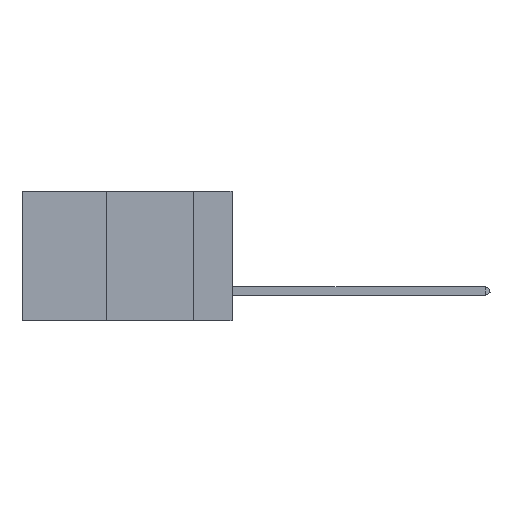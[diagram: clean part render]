
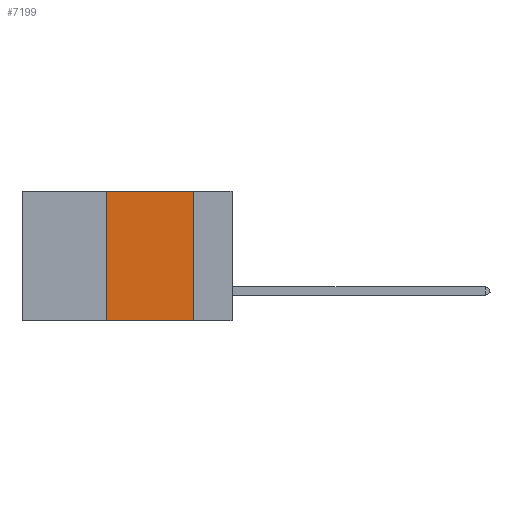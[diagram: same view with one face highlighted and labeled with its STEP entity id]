
A CAD part, left-side view. The second image highlights one B-rep face of the part: STEP entity #7199.
In plain terms, the highlighted planar face has unit normal (-1, 0, 0).
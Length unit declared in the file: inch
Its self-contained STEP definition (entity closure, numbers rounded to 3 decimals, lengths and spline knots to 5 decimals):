
#320 = CARTESIAN_POINT ( 'NONE',  ( 0., 0.36, -0.37 ) ) ;
#374 = PLANE ( 'NONE',  #565 ) ;
#406 = EDGE_CURVE ( 'NONE', #9593, #12803, #15232, .T. ) ;
#565 = AXIS2_PLACEMENT_3D ( 'NONE', #4045, #9053, #6343 ) ;
#1202 = LINE ( 'NONE', #9363, #12436 ) ;
#2927 = VECTOR ( 'NONE', #4506, 39.37008 ) ;
#2974 = EDGE_CURVE ( 'NONE', #14182, #14247, #10661, .T. ) ;
#3828 = ORIENTED_EDGE ( 'NONE', *, *, #2974, .T. ) ;
#4045 = CARTESIAN_POINT ( 'NONE',  ( 0., 0.6, 0. ) ) ;
#4506 = DIRECTION ( 'NONE',  ( 0., -1., 0. ) ) ;
#4891 = FACE_OUTER_BOUND ( 'NONE', #14058, .T. ) ;
#6343 = DIRECTION ( 'NONE',  ( 0., 0., -1. ) ) ;
#7199 = ADVANCED_FACE ( 'NONE', ( #4891 ), #374, .F. ) ;
#7297 = DIRECTION ( 'NONE',  ( 0., 0., 1. ) ) ;
#8455 = EDGE_CURVE ( 'NONE', #12803, #14247, #1202, .T. ) ;
#8496 = ORIENTED_EDGE ( 'NONE', *, *, #9040, .F. ) ;
#9029 = DIRECTION ( 'NONE',  ( 0., -1., 0. ) ) ;
#9040 = EDGE_CURVE ( 'NONE', #14182, #9593, #13275, .T. ) ;
#9053 = DIRECTION ( 'NONE',  ( 1., 0., 0. ) ) ;
#9363 = CARTESIAN_POINT ( 'NONE',  ( 0., 0.11, 0. ) ) ;
#9369 = CARTESIAN_POINT ( 'NONE',  ( 0., 0.11, 0. ) ) ;
#9593 = VERTEX_POINT ( 'NONE', #15968 ) ;
#9662 = ORIENTED_EDGE ( 'NONE', *, *, #406, .F. ) ;
#10661 = LINE ( 'NONE', #10791, #2927 ) ;
#10791 = CARTESIAN_POINT ( 'NONE',  ( 0., 0.6, -0.37 ) ) ;
#11716 = CARTESIAN_POINT ( 'NONE',  ( 0., 0.11, -0.37 ) ) ;
#12436 = VECTOR ( 'NONE', #12912, 39.37008 ) ;
#12686 = VECTOR ( 'NONE', #9029, 39.37008 ) ;
#12774 = CARTESIAN_POINT ( 'NONE',  ( 0., 0.6, 0. ) ) ;
#12803 = VERTEX_POINT ( 'NONE', #9369 ) ;
#12912 = DIRECTION ( 'NONE',  ( 0., 0., -1. ) ) ;
#13275 = LINE ( 'NONE', #14936, #15795 ) ;
#14058 = EDGE_LOOP ( 'NONE', ( #14689, #9662, #8496, #3828 ) ) ;
#14182 = VERTEX_POINT ( 'NONE', #320 ) ;
#14247 = VERTEX_POINT ( 'NONE', #11716 ) ;
#14689 = ORIENTED_EDGE ( 'NONE', *, *, #8455, .F. ) ;
#14936 = CARTESIAN_POINT ( 'NONE',  ( 0., 0.36, 0. ) ) ;
#15232 = LINE ( 'NONE', #12774, #12686 ) ;
#15795 = VECTOR ( 'NONE', #7297, 39.37008 ) ;
#15968 = CARTESIAN_POINT ( 'NONE',  ( 0., 0.36, 0. ) ) ;
